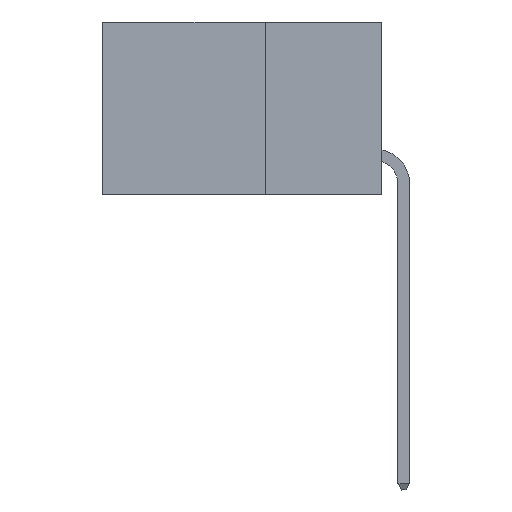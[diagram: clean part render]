
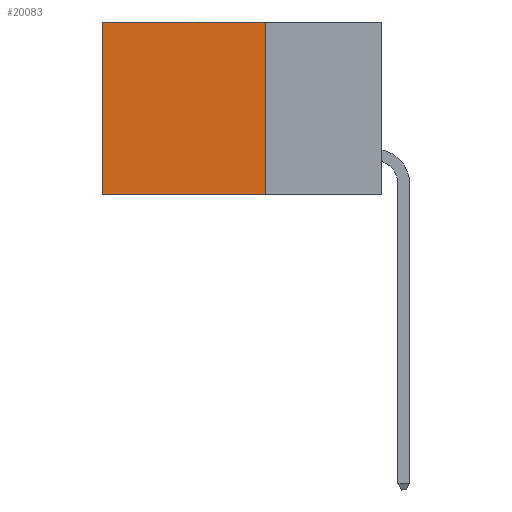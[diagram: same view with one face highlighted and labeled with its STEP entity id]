
A CAD part, left-side view. The second image highlights one B-rep face of the part: STEP entity #20083.
In plain terms, the highlighted planar face has unit normal (-1, 0, 0).
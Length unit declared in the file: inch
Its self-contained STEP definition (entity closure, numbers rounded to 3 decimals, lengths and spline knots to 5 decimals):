
#16 = CARTESIAN_POINT ( 'NONE',  ( 0.2875, 0.6, 0. ) ) ;
#1767 = ORIENTED_EDGE ( 'NONE', *, *, #4586, .F. ) ;
#1915 = ORIENTED_EDGE ( 'NONE', *, *, #47273, .F. ) ;
#2550 = LINE ( 'NONE', #24356, #35302 ) ;
#3962 = DIRECTION ( 'NONE',  ( 0., 1., 0. ) ) ;
#4586 = EDGE_CURVE ( 'NONE', #8882, #40677, #2550, .T. ) ;
#5468 = EDGE_CURVE ( 'NONE', #25205, #37633, #23553, .T. ) ;
#6094 = CARTESIAN_POINT ( 'NONE',  ( 0.2875, 0.25, 0. ) ) ;
#6144 = EDGE_CURVE ( 'NONE', #37633, #40677, #25199, .T. ) ;
#6260 = DIRECTION ( 'NONE',  ( 0., 0., -1. ) ) ;
#6356 = DIRECTION ( 'NONE',  ( 0., 0., -1. ) ) ;
#6722 = CARTESIAN_POINT ( 'NONE',  ( 0.2875, 0.25, -0.37 ) ) ;
#7699 = DIRECTION ( 'NONE',  ( 0., 0., -1. ) ) ;
#8882 = VERTEX_POINT ( 'NONE', #6722 ) ;
#9543 = EDGE_LOOP ( 'NONE', ( #21072, #1767, #1915, #30448 ) ) ;
#11883 = VECTOR ( 'NONE', #3962, 39.37008 ) ;
#12899 = VECTOR ( 'NONE', #7699, 39.37008 ) ;
#14776 = CARTESIAN_POINT ( 'NONE',  ( 0.2875, 0.6, 0. ) ) ;
#18050 = PLANE ( 'NONE',  #18310 ) ;
#18310 = AXIS2_PLACEMENT_3D ( 'NONE', #6094, #29006, #6260 ) ;
#20083 = ADVANCED_FACE ( 'NONE', ( #35889 ), #18050, .F. ) ;
#20589 = DIRECTION ( 'NONE',  ( 0., 1., 0. ) ) ;
#21072 = ORIENTED_EDGE ( 'NONE', *, *, #6144, .T. ) ;
#23443 = CARTESIAN_POINT ( 'NONE',  ( 0.2875, 0.25, 0. ) ) ;
#23553 = LINE ( 'NONE', #25911, #11883 ) ;
#24356 = CARTESIAN_POINT ( 'NONE',  ( 0.2875, 0.25, -0.37 ) ) ;
#25199 = LINE ( 'NONE', #14776, #12899 ) ;
#25205 = VERTEX_POINT ( 'NONE', #23443 ) ;
#25911 = CARTESIAN_POINT ( 'NONE',  ( 0.2875, 0.25, 0. ) ) ;
#29006 = DIRECTION ( 'NONE',  ( 1., 0., 0. ) ) ;
#30448 = ORIENTED_EDGE ( 'NONE', *, *, #5468, .T. ) ;
#35302 = VECTOR ( 'NONE', #20589, 39.37008 ) ;
#35889 = FACE_OUTER_BOUND ( 'NONE', #9543, .T. ) ;
#37538 = CARTESIAN_POINT ( 'NONE',  ( 0.2875, 0.6, -0.37 ) ) ;
#37633 = VERTEX_POINT ( 'NONE', #16 ) ;
#39879 = CARTESIAN_POINT ( 'NONE',  ( 0.2875, 0.25, 0. ) ) ;
#40677 = VERTEX_POINT ( 'NONE', #37538 ) ;
#43150 = LINE ( 'NONE', #39879, #43760 ) ;
#43760 = VECTOR ( 'NONE', #6356, 39.37008 ) ;
#47273 = EDGE_CURVE ( 'NONE', #25205, #8882, #43150, .T. ) ;
